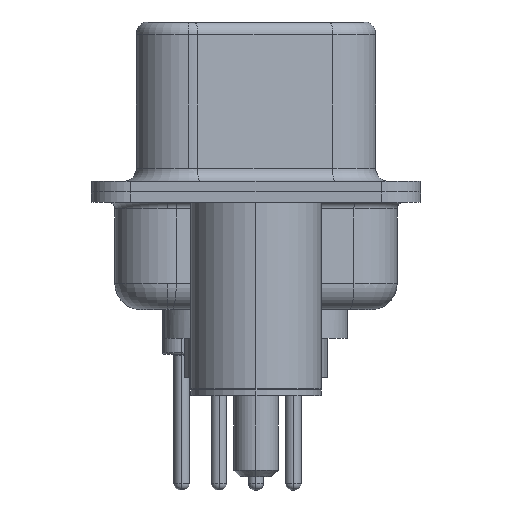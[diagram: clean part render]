
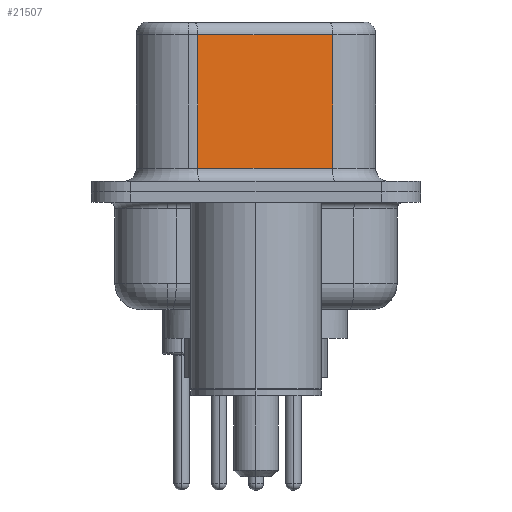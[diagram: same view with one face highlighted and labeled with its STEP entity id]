
A CAD part, left-side view. The second image highlights one B-rep face of the part: STEP entity #21507.
In plain terms, the highlighted planar face has unit normal (-0.985, -0.174, 0).
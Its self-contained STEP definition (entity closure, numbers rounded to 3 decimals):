
#87 = VECTOR ( 'NONE', #15543, 1000. ) ;
#608 = CARTESIAN_POINT ( 'NONE',  ( 4.585, -2.927, 6.02 ) ) ;
#929 = CARTESIAN_POINT ( 'NONE',  ( 3.675, 2.233, 6.02 ) ) ;
#1273 = VERTEX_POINT ( 'NONE', #2628 ) ;
#1884 = PLANE ( 'NONE',  #9551 ) ;
#2628 = CARTESIAN_POINT ( 'NONE',  ( 3.675, 2.233, 0.9 ) ) ;
#3137 = LINE ( 'NONE', #7867, #15963 ) ;
#3816 = CARTESIAN_POINT ( 'NONE',  ( 4.585, -2.927, 6.52 ) ) ;
#5570 = CARTESIAN_POINT ( 'NONE',  ( 3.675, 2.233, 6.52 ) ) ;
#5867 = DIRECTION ( 'NONE',  ( 0., 0., -1. ) ) ;
#6945 = LINE ( 'NONE', #5570, #12004 ) ;
#7659 = EDGE_CURVE ( 'NONE', #21122, #23858, #9320, .T. ) ;
#7867 = CARTESIAN_POINT ( 'NONE',  ( 4.585, -2.927, 6.52 ) ) ;
#7977 = EDGE_CURVE ( 'NONE', #23858, #1273, #6945, .T. ) ;
#9320 = LINE ( 'NONE', #15176, #17681 ) ;
#9489 = DIRECTION ( 'NONE',  ( 0., 0., -1. ) ) ;
#9551 = AXIS2_PLACEMENT_3D ( 'NONE', #3816, #17151, #23034 ) ;
#12004 = VECTOR ( 'NONE', #9489, 1000. ) ;
#14460 = CARTESIAN_POINT ( 'NONE',  ( 4.585, -2.927, 0.9 ) ) ;
#15176 = CARTESIAN_POINT ( 'NONE',  ( 4.585, -2.927, 6.02 ) ) ;
#15543 = DIRECTION ( 'NONE',  ( 0.174, -0.985, 0. ) ) ;
#15752 = ORIENTED_EDGE ( 'NONE', *, *, #22717, .F. ) ;
#15963 = VECTOR ( 'NONE', #5867, 1000. ) ;
#16198 = CARTESIAN_POINT ( 'NONE',  ( 4.585, -2.927, 0.9 ) ) ;
#16378 = ORIENTED_EDGE ( 'NONE', *, *, #7977, .T. ) ;
#17134 = ORIENTED_EDGE ( 'NONE', *, *, #7659, .T. ) ;
#17151 = DIRECTION ( 'NONE',  ( 0.985, 0.174, 0. ) ) ;
#17681 = VECTOR ( 'NONE', #20801, 1000. ) ;
#18365 = LINE ( 'NONE', #14460, #87 ) ;
#18773 = FACE_OUTER_BOUND ( 'NONE', #22070, .T. ) ;
#19032 = ORIENTED_EDGE ( 'NONE', *, *, #22880, .T. ) ;
#20801 = DIRECTION ( 'NONE',  ( -0.174, 0.985, 0. ) ) ;
#21122 = VERTEX_POINT ( 'NONE', #608 ) ;
#21507 = ADVANCED_FACE ( 'NONE', ( #18773 ), #1884, .F. ) ;
#22070 = EDGE_LOOP ( 'NONE', ( #15752, #17134, #16378, #19032 ) ) ;
#22717 = EDGE_CURVE ( 'NONE', #21122, #24204, #3137, .T. ) ;
#22880 = EDGE_CURVE ( 'NONE', #1273, #24204, #18365, .T. ) ;
#23034 = DIRECTION ( 'NONE',  ( -0.174, 0.985, 0. ) ) ;
#23858 = VERTEX_POINT ( 'NONE', #929 ) ;
#24204 = VERTEX_POINT ( 'NONE', #16198 ) ;
